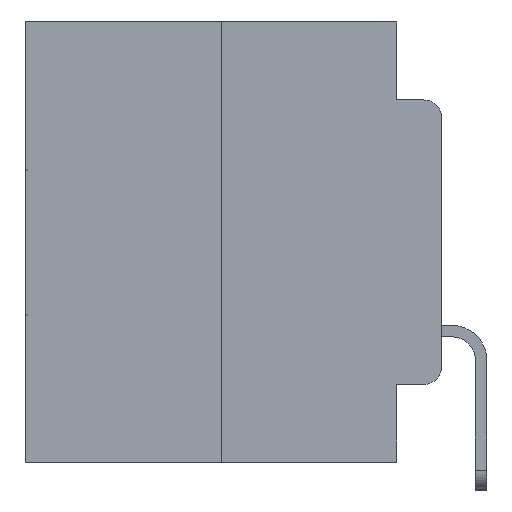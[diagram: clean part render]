
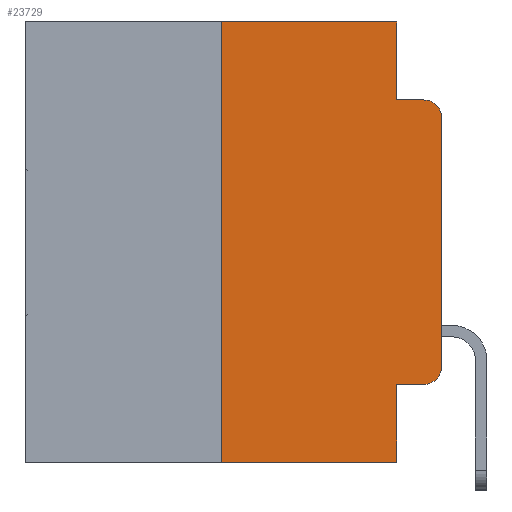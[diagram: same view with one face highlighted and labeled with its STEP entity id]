
A CAD part, left-side view. The second image highlights one B-rep face of the part: STEP entity #23729.
In plain terms, the highlighted planar face has unit normal (-1, 0, 0).
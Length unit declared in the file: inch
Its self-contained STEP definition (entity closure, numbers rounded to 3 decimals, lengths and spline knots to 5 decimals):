
#633 = VECTOR ( 'NONE', #3719, 39.37008 ) ;
#777 = EDGE_CURVE ( 'NONE', #13281, #11630, #6979, .T. ) ;
#1067 = LINE ( 'NONE', #7831, #12871 ) ;
#1123 = CARTESIAN_POINT ( 'NONE',  ( 0., 0.051, -0.4115 ) ) ;
#1196 = CARTESIAN_POINT ( 'NONE',  ( 0., 0.051, -0.4115 ) ) ;
#1248 = ORIENTED_EDGE ( 'NONE', *, *, #14773, .F. ) ;
#1293 = DIRECTION ( 'NONE',  ( 1., 0., 0. ) ) ;
#3245 = DIRECTION ( 'NONE',  ( -1., 0., 0. ) ) ;
#3423 = ORIENTED_EDGE ( 'NONE', *, *, #4653, .F. ) ;
#3719 = DIRECTION ( 'NONE',  ( 0., 0., -1. ) ) ;
#3816 = ORIENTED_EDGE ( 'NONE', *, *, #24837, .F. ) ;
#3911 = ORIENTED_EDGE ( 'NONE', *, *, #777, .F. ) ;
#4653 = EDGE_CURVE ( 'NONE', #27918, #22291, #20967, .T. ) ;
#5363 = AXIS2_PLACEMENT_3D ( 'NONE', #17532, #1293, #17630 ) ;
#5423 = CARTESIAN_POINT ( 'NONE',  ( 0., 0.25, 0. ) ) ;
#5436 = VECTOR ( 'NONE', #13075, 39.37008 ) ;
#5658 = ORIENTED_EDGE ( 'NONE', *, *, #23061, .T. ) ;
#6838 = VECTOR ( 'NONE', #23449, 39.37008 ) ;
#6979 = LINE ( 'NONE', #21915, #633 ) ;
#7225 = CARTESIAN_POINT ( 'NONE',  ( 0., 0., -0.1085 ) ) ;
#7331 = LINE ( 'NONE', #1123, #24867 ) ;
#7466 = CARTESIAN_POINT ( 'NONE',  ( 0., 0.473, -0.5 ) ) ;
#7831 = CARTESIAN_POINT ( 'NONE',  ( 0., 0.473, 0. ) ) ;
#8079 = CARTESIAN_POINT ( 'NONE',  ( 0., 0., 0. ) ) ;
#8266 = PLANE ( 'NONE',  #5363 ) ;
#8351 = EDGE_CURVE ( 'NONE', #12132, #29790, #11153, .T. ) ;
#8736 = AXIS2_PLACEMENT_3D ( 'NONE', #9481, #25440, #11846 ) ;
#8815 = VECTOR ( 'NONE', #13060, 39.37008 ) ;
#9481 = CARTESIAN_POINT ( 'NONE',  ( 0., 0.02, -0.3915 ) ) ;
#9818 = ORIENTED_EDGE ( 'NONE', *, *, #8351, .T. ) ;
#9955 = CARTESIAN_POINT ( 'NONE',  ( 0., 0.051, -0.0885 ) ) ;
#10110 = DIRECTION ( 'NONE',  ( 0., 0., 1. ) ) ;
#10166 = DIRECTION ( 'NONE',  ( 0., -1., 0. ) ) ;
#10498 = EDGE_CURVE ( 'NONE', #12264, #12537, #1067, .T. ) ;
#11025 = CARTESIAN_POINT ( 'NONE',  ( 0., 0.051, -0.5 ) ) ;
#11026 = VECTOR ( 'NONE', #24049, 39.37008 ) ;
#11153 = CIRCLE ( 'NONE', #8736, 0.02 ) ;
#11183 = ORIENTED_EDGE ( 'NONE', *, *, #10498, .F. ) ;
#11630 = VERTEX_POINT ( 'NONE', #11025 ) ;
#11846 = DIRECTION ( 'NONE',  ( 0., 0., -1. ) ) ;
#12132 = VERTEX_POINT ( 'NONE', #15610 ) ;
#12264 = VERTEX_POINT ( 'NONE', #15989 ) ;
#12537 = VERTEX_POINT ( 'NONE', #23884 ) ;
#12741 = CIRCLE ( 'NONE', #20137, 0.02 ) ;
#12820 = FACE_OUTER_BOUND ( 'NONE', #13316, .T. ) ;
#12871 = VECTOR ( 'NONE', #10166, 39.37008 ) ;
#13060 = DIRECTION ( 'NONE',  ( 0., -1., 0. ) ) ;
#13075 = DIRECTION ( 'NONE',  ( 0., 0., -1. ) ) ;
#13281 = VERTEX_POINT ( 'NONE', #1196 ) ;
#13316 = EDGE_LOOP ( 'NONE', ( #22494, #22164, #3423, #3816, #11183, #1248, #26590, #3911, #5658, #9818 ) ) ;
#13845 = EDGE_CURVE ( 'NONE', #18126, #22291, #12741, .T. ) ;
#14684 = EDGE_CURVE ( 'NONE', #20947, #11630, #18369, .T. ) ;
#14773 = EDGE_CURVE ( 'NONE', #20947, #12264, #22232, .T. ) ;
#14811 = CARTESIAN_POINT ( 'NONE',  ( 0., 0., -0.3915 ) ) ;
#15522 = VECTOR ( 'NONE', #10110, 39.37008 ) ;
#15610 = CARTESIAN_POINT ( 'NONE',  ( 0., 0.02, -0.4115 ) ) ;
#15989 = CARTESIAN_POINT ( 'NONE',  ( 0., 0.25, 0. ) ) ;
#16787 = LINE ( 'NONE', #8079, #11026 ) ;
#17191 = CARTESIAN_POINT ( 'NONE',  ( 0., 0.02, -0.1085 ) ) ;
#17532 = CARTESIAN_POINT ( 'NONE',  ( 0., 0.473, 0. ) ) ;
#17630 = DIRECTION ( 'NONE',  ( 0., 0., -1. ) ) ;
#18126 = VERTEX_POINT ( 'NONE', #7225 ) ;
#18202 = CARTESIAN_POINT ( 'NONE',  ( 0., 0.02, -0.0885 ) ) ;
#18369 = LINE ( 'NONE', #7466, #6838 ) ;
#19448 = DIRECTION ( 'NONE',  ( 0., 0., -1. ) ) ;
#19788 = EDGE_CURVE ( 'NONE', #29790, #18126, #16787, .T. ) ;
#20137 = AXIS2_PLACEMENT_3D ( 'NONE', #17191, #3245, #19448 ) ;
#20947 = VERTEX_POINT ( 'NONE', #28595 ) ;
#20967 = LINE ( 'NONE', #28749, #8815 ) ;
#21915 = CARTESIAN_POINT ( 'NONE',  ( 0., 0.051, 0. ) ) ;
#22164 = ORIENTED_EDGE ( 'NONE', *, *, #13845, .T. ) ;
#22232 = LINE ( 'NONE', #5423, #15522 ) ;
#22291 = VERTEX_POINT ( 'NONE', #18202 ) ;
#22494 = ORIENTED_EDGE ( 'NONE', *, *, #19788, .T. ) ;
#22992 = LINE ( 'NONE', #26632, #5436 ) ;
#23061 = EDGE_CURVE ( 'NONE', #13281, #12132, #7331, .T. ) ;
#23449 = DIRECTION ( 'NONE',  ( 0., -1., 0. ) ) ;
#23729 = ADVANCED_FACE ( 'NONE', ( #12820 ), #8266, .F. ) ;
#23884 = CARTESIAN_POINT ( 'NONE',  ( 0., 0.051, 0. ) ) ;
#24049 = DIRECTION ( 'NONE',  ( 0., 0., 1. ) ) ;
#24170 = DIRECTION ( 'NONE',  ( 0., -1., 0. ) ) ;
#24837 = EDGE_CURVE ( 'NONE', #12537, #27918, #22992, .T. ) ;
#24867 = VECTOR ( 'NONE', #24170, 39.37008 ) ;
#25440 = DIRECTION ( 'NONE',  ( -1., 0., 0. ) ) ;
#26590 = ORIENTED_EDGE ( 'NONE', *, *, #14684, .T. ) ;
#26632 = CARTESIAN_POINT ( 'NONE',  ( 0., 0.051, 0. ) ) ;
#27918 = VERTEX_POINT ( 'NONE', #9955 ) ;
#28595 = CARTESIAN_POINT ( 'NONE',  ( 0., 0.25, -0.5 ) ) ;
#28749 = CARTESIAN_POINT ( 'NONE',  ( 0., 0.051, -0.0885 ) ) ;
#29790 = VERTEX_POINT ( 'NONE', #14811 ) ;
